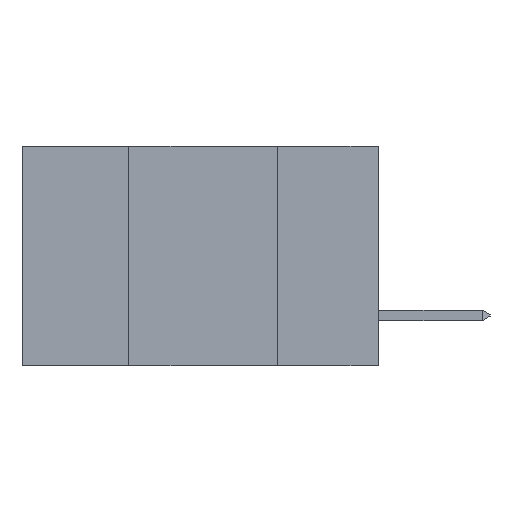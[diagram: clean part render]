
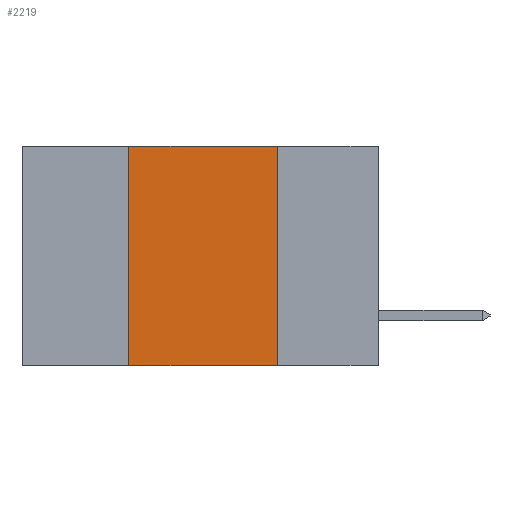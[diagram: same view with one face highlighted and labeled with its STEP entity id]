
A CAD part, left-side view. The second image highlights one B-rep face of the part: STEP entity #2219.
In plain terms, the highlighted planar face has unit normal (-1, 0, 0).
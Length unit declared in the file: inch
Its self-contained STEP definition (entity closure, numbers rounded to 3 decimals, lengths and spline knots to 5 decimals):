
#13 = ORIENTED_EDGE ( 'NONE', *, *, #12800, .F. ) ;
#134 = VECTOR ( 'NONE', #5829, 39.37008 ) ;
#172 = CARTESIAN_POINT ( 'NONE',  ( 0., 0.17, -0.37 ) ) ;
#322 = CARTESIAN_POINT ( 'NONE',  ( 0., 0.42, -0.37 ) ) ;
#607 = DIRECTION ( 'NONE',  ( 1., 0., 0. ) ) ;
#1636 = VERTEX_POINT ( 'NONE', #322 ) ;
#2219 = ADVANCED_FACE ( 'NONE', ( #11256 ), #3282, .F. ) ;
#2812 = CARTESIAN_POINT ( 'NONE',  ( 0., 0.6, -0.37 ) ) ;
#3282 = PLANE ( 'NONE',  #11545 ) ;
#3673 = CARTESIAN_POINT ( 'NONE',  ( 0., 0.6, 0. ) ) ;
#4108 = CARTESIAN_POINT ( 'NONE',  ( 0., 0.6, 0. ) ) ;
#4489 = CARTESIAN_POINT ( 'NONE',  ( 0., 0.17, -0.37 ) ) ;
#4808 = VERTEX_POINT ( 'NONE', #172 ) ;
#4878 = VERTEX_POINT ( 'NONE', #16746 ) ;
#5212 = LINE ( 'NONE', #4108, #8317 ) ;
#5305 = ORIENTED_EDGE ( 'NONE', *, *, #13670, .F. ) ;
#5829 = DIRECTION ( 'NONE',  ( 0., 0., -1. ) ) ;
#6162 = VECTOR ( 'NONE', #14735, 39.37008 ) ;
#6292 = LINE ( 'NONE', #7776, #9394 ) ;
#7776 = CARTESIAN_POINT ( 'NONE',  ( 0., 0.42, -0.37 ) ) ;
#8317 = VECTOR ( 'NONE', #10747, 39.37008 ) ;
#8571 = ORIENTED_EDGE ( 'NONE', *, *, #9268, .T. ) ;
#9268 = EDGE_CURVE ( 'NONE', #1636, #4808, #10087, .T. ) ;
#9394 = VECTOR ( 'NONE', #15540, 39.37008 ) ;
#10087 = LINE ( 'NONE', #2812, #6162 ) ;
#10747 = DIRECTION ( 'NONE',  ( 0., -1., 0. ) ) ;
#10982 = LINE ( 'NONE', #4489, #134 ) ;
#11042 = EDGE_CURVE ( 'NONE', #1636, #12515, #6292, .T. ) ;
#11256 = FACE_OUTER_BOUND ( 'NONE', #16108, .T. ) ;
#11545 = AXIS2_PLACEMENT_3D ( 'NONE', #3673, #607, #16632 ) ;
#12488 = ORIENTED_EDGE ( 'NONE', *, *, #11042, .F. ) ;
#12515 = VERTEX_POINT ( 'NONE', #15381 ) ;
#12800 = EDGE_CURVE ( 'NONE', #12515, #4878, #5212, .T. ) ;
#13670 = EDGE_CURVE ( 'NONE', #4878, #4808, #10982, .T. ) ;
#14735 = DIRECTION ( 'NONE',  ( 0., -1., 0. ) ) ;
#15381 = CARTESIAN_POINT ( 'NONE',  ( 0., 0.42, 0. ) ) ;
#15540 = DIRECTION ( 'NONE',  ( 0., 0., 1. ) ) ;
#16108 = EDGE_LOOP ( 'NONE', ( #5305, #13, #12488, #8571 ) ) ;
#16632 = DIRECTION ( 'NONE',  ( 0., 0., -1. ) ) ;
#16746 = CARTESIAN_POINT ( 'NONE',  ( 0., 0.17, 0. ) ) ;
